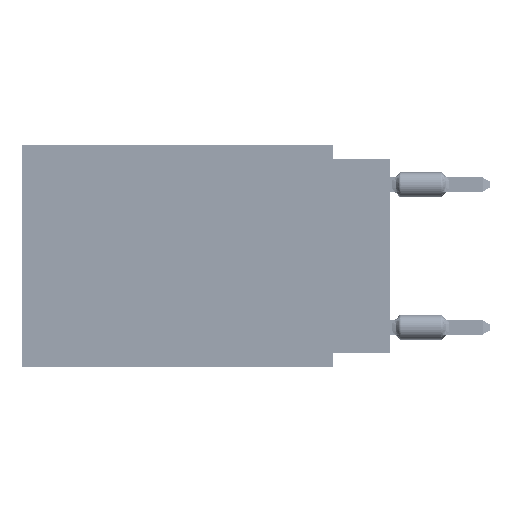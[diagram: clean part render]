
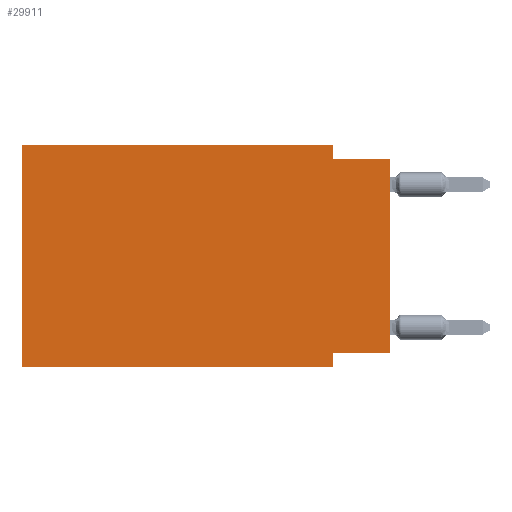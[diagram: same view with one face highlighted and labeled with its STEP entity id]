
A CAD part, left-side view. The second image highlights one B-rep face of the part: STEP entity #29911.
In plain terms, the highlighted planar face has unit normal (-1, 0, 0).
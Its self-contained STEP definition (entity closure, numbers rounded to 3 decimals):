
#351 = EDGE_CURVE ( 'NONE', #8154, #66137, #26912, .T. ) ;
#3614 = LINE ( 'NONE', #60065, #26441 ) ;
#4364 = ORIENTED_EDGE ( 'NONE', *, *, #26966, .F. ) ;
#6791 = VECTOR ( 'NONE', #27838, 1000. ) ;
#7004 = LINE ( 'NONE', #63123, #6791 ) ;
#7249 = CARTESIAN_POINT ( 'NONE',  ( 0., 2.54, -9.906 ) ) ;
#7577 = LINE ( 'NONE', #7249, #64666 ) ;
#7760 = ORIENTED_EDGE ( 'NONE', *, *, #28554, .T. ) ;
#8154 = VERTEX_POINT ( 'NONE', #56557 ) ;
#10252 = LINE ( 'NONE', #25359, #44696 ) ;
#10334 = PLANE ( 'NONE',  #18890 ) ;
#14032 = DIRECTION ( 'NONE',  ( 0., -1., 0. ) ) ;
#14707 = ORIENTED_EDGE ( 'NONE', *, *, #18432, .F. ) ;
#14979 = CARTESIAN_POINT ( 'NONE',  ( 0., 0., -0.635 ) ) ;
#17071 = CARTESIAN_POINT ( 'NONE',  ( 0., 16.383, 0. ) ) ;
#18432 = EDGE_CURVE ( 'NONE', #22864, #38629, #7577, .T. ) ;
#18890 = AXIS2_PLACEMENT_3D ( 'NONE', #35526, #66107, #56024 ) ;
#18913 = CARTESIAN_POINT ( 'NONE',  ( 0., 2.54, -9.271 ) ) ;
#19220 = CARTESIAN_POINT ( 'NONE',  ( 0., 16.383, -9.906 ) ) ;
#21623 = EDGE_CURVE ( 'NONE', #27663, #25283, #35441, .T. ) ;
#22864 = VERTEX_POINT ( 'NONE', #18913 ) ;
#23407 = CARTESIAN_POINT ( 'NONE',  ( 0., 16.383, 0. ) ) ;
#25283 = VERTEX_POINT ( 'NONE', #23407 ) ;
#25359 = CARTESIAN_POINT ( 'NONE',  ( 0., 0., -9.271 ) ) ;
#25613 = EDGE_CURVE ( 'NONE', #39970, #30130, #26725, .T. ) ;
#26441 = VECTOR ( 'NONE', #14032, 1000. ) ;
#26725 = LINE ( 'NONE', #41823, #30959 ) ;
#26912 = LINE ( 'NONE', #63187, #59136 ) ;
#26966 = EDGE_CURVE ( 'NONE', #25283, #39970, #63117, .T. ) ;
#27663 = VERTEX_POINT ( 'NONE', #19220 ) ;
#27838 = DIRECTION ( 'NONE',  ( 0., -1., 0. ) ) ;
#28554 = EDGE_CURVE ( 'NONE', #27663, #38629, #3614, .T. ) ;
#29265 = CARTESIAN_POINT ( 'NONE',  ( 0., 2.54, 0. ) ) ;
#29911 = ADVANCED_FACE ( 'NONE', ( #40558 ), #10334, .F. ) ;
#30130 = VERTEX_POINT ( 'NONE', #52980 ) ;
#30358 = EDGE_CURVE ( 'NONE', #8154, #22864, #10252, .T. ) ;
#30959 = VECTOR ( 'NONE', #46875, 1000. ) ;
#35441 = LINE ( 'NONE', #41454, #48752 ) ;
#35526 = CARTESIAN_POINT ( 'NONE',  ( 0., 16.383, 0. ) ) ;
#37176 = ORIENTED_EDGE ( 'NONE', *, *, #30358, .F. ) ;
#38629 = VERTEX_POINT ( 'NONE', #58180 ) ;
#39970 = VERTEX_POINT ( 'NONE', #29265 ) ;
#40558 = FACE_OUTER_BOUND ( 'NONE', #59332, .T. ) ;
#41135 = DIRECTION ( 'NONE',  ( 0., 1., 0. ) ) ;
#41454 = CARTESIAN_POINT ( 'NONE',  ( 0., 16.383, 0. ) ) ;
#41823 = CARTESIAN_POINT ( 'NONE',  ( 0., 2.54, 0. ) ) ;
#42332 = DIRECTION ( 'NONE',  ( 0., 0., 1. ) ) ;
#43524 = DIRECTION ( 'NONE',  ( 0., 0., -1. ) ) ;
#44696 = VECTOR ( 'NONE', #41135, 1000. ) ;
#46419 = ORIENTED_EDGE ( 'NONE', *, *, #351, .T. ) ;
#46875 = DIRECTION ( 'NONE',  ( 0., 0., -1. ) ) ;
#47525 = ORIENTED_EDGE ( 'NONE', *, *, #53800, .F. ) ;
#48752 = VECTOR ( 'NONE', #66026, 1000. ) ;
#49892 = VECTOR ( 'NONE', #52698, 1000. ) ;
#52698 = DIRECTION ( 'NONE',  ( 0., -1., 0. ) ) ;
#52980 = CARTESIAN_POINT ( 'NONE',  ( 0., 2.54, -0.635 ) ) ;
#53800 = EDGE_CURVE ( 'NONE', #30130, #66137, #7004, .T. ) ;
#56024 = DIRECTION ( 'NONE',  ( 0., 0., -1. ) ) ;
#56557 = CARTESIAN_POINT ( 'NONE',  ( 0., 0., -9.271 ) ) ;
#58180 = CARTESIAN_POINT ( 'NONE',  ( 0., 2.54, -9.906 ) ) ;
#59136 = VECTOR ( 'NONE', #42332, 1000. ) ;
#59332 = EDGE_LOOP ( 'NONE', ( #46419, #47525, #65171, #4364, #66418, #7760, #14707, #37176 ) ) ;
#60065 = CARTESIAN_POINT ( 'NONE',  ( 0., 16.383, -9.906 ) ) ;
#63117 = LINE ( 'NONE', #17071, #49892 ) ;
#63123 = CARTESIAN_POINT ( 'NONE',  ( 0., 0., -0.635 ) ) ;
#63187 = CARTESIAN_POINT ( 'NONE',  ( 0., 0., 0. ) ) ;
#64666 = VECTOR ( 'NONE', #43524, 1000. ) ;
#65171 = ORIENTED_EDGE ( 'NONE', *, *, #25613, .F. ) ;
#66026 = DIRECTION ( 'NONE',  ( 0., 0., 1. ) ) ;
#66107 = DIRECTION ( 'NONE',  ( 1., 0., 0. ) ) ;
#66137 = VERTEX_POINT ( 'NONE', #14979 ) ;
#66418 = ORIENTED_EDGE ( 'NONE', *, *, #21623, .F. ) ;
